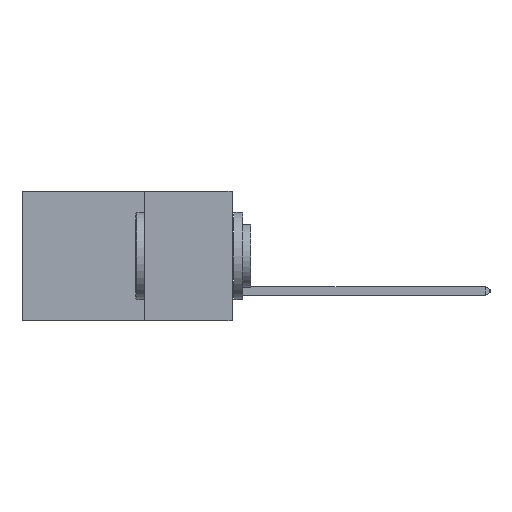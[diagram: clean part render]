
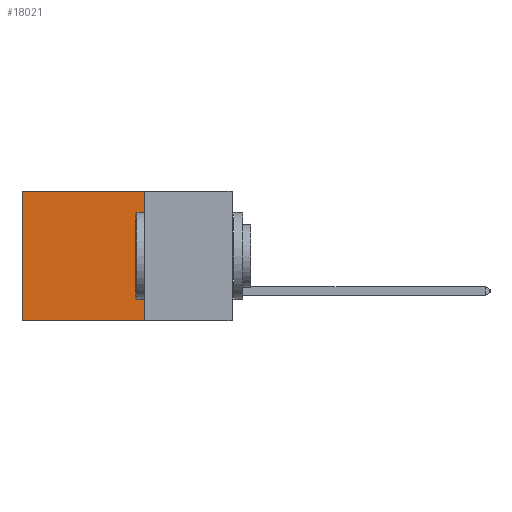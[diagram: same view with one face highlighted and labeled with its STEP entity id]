
A CAD part, left-side view. The second image highlights one B-rep face of the part: STEP entity #18021.
In plain terms, the highlighted planar face has unit normal (-1, 0, 0).
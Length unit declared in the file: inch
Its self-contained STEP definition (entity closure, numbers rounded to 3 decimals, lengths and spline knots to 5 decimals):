
#909 = LINE ( 'NONE', #10781, #17000 ) ;
#1074 = CARTESIAN_POINT ( 'NONE',  ( 0.2875, 0.25, -0.37 ) ) ;
#1307 = LINE ( 'NONE', #15638, #10499 ) ;
#1775 = CARTESIAN_POINT ( 'NONE',  ( 0.2875, 0.25, 0. ) ) ;
#2043 = EDGE_CURVE ( 'NONE', #9219, #10675, #909, .T. ) ;
#3109 = VECTOR ( 'NONE', #16447, 39.37008 ) ;
#3389 = LINE ( 'NONE', #11579, #20057 ) ;
#4572 = VERTEX_POINT ( 'NONE', #12360 ) ;
#5770 = DIRECTION ( 'NONE',  ( 0., 0., -1. ) ) ;
#5886 = FACE_OUTER_BOUND ( 'NONE', #11552, .T. ) ;
#6173 = CARTESIAN_POINT ( 'NONE',  ( 0.2875, 0.6, -0.37 ) ) ;
#6314 = ORIENTED_EDGE ( 'NONE', *, *, #9145, .T. ) ;
#6659 = CARTESIAN_POINT ( 'NONE',  ( 0.2875, 0.25, 0. ) ) ;
#6935 = LINE ( 'NONE', #6659, #3109 ) ;
#7528 = AXIS2_PLACEMENT_3D ( 'NONE', #17441, #7693, #18992 ) ;
#7589 = VERTEX_POINT ( 'NONE', #1775 ) ;
#7693 = DIRECTION ( 'NONE',  ( 1., 0., 0. ) ) ;
#9145 = EDGE_CURVE ( 'NONE', #4572, #10675, #1307, .T. ) ;
#9219 = VERTEX_POINT ( 'NONE', #1074 ) ;
#9742 = ORIENTED_EDGE ( 'NONE', *, *, #14224, .F. ) ;
#10499 = VECTOR ( 'NONE', #5770, 39.37008 ) ;
#10631 = DIRECTION ( 'NONE',  ( 0., 1., 0. ) ) ;
#10675 = VERTEX_POINT ( 'NONE', #6173 ) ;
#10725 = ORIENTED_EDGE ( 'NONE', *, *, #2043, .F. ) ;
#10781 = CARTESIAN_POINT ( 'NONE',  ( 0.2875, 0.25, -0.37 ) ) ;
#11552 = EDGE_LOOP ( 'NONE', ( #6314, #10725, #9742, #16364 ) ) ;
#11579 = CARTESIAN_POINT ( 'NONE',  ( 0.2875, 0.25, 0. ) ) ;
#12360 = CARTESIAN_POINT ( 'NONE',  ( 0.2875, 0.6, 0. ) ) ;
#12570 = PLANE ( 'NONE',  #7528 ) ;
#13287 = DIRECTION ( 'NONE',  ( 0., 0., -1. ) ) ;
#14224 = EDGE_CURVE ( 'NONE', #7589, #9219, #3389, .T. ) ;
#14924 = EDGE_CURVE ( 'NONE', #7589, #4572, #6935, .T. ) ;
#15638 = CARTESIAN_POINT ( 'NONE',  ( 0.2875, 0.6, 0. ) ) ;
#16364 = ORIENTED_EDGE ( 'NONE', *, *, #14924, .T. ) ;
#16447 = DIRECTION ( 'NONE',  ( 0., 1., 0. ) ) ;
#17000 = VECTOR ( 'NONE', #10631, 39.37008 ) ;
#17441 = CARTESIAN_POINT ( 'NONE',  ( 0.2875, 0.25, 0. ) ) ;
#18021 = ADVANCED_FACE ( 'NONE', ( #5886 ), #12570, .F. ) ;
#18992 = DIRECTION ( 'NONE',  ( 0., 0., -1. ) ) ;
#20057 = VECTOR ( 'NONE', #13287, 39.37008 ) ;
